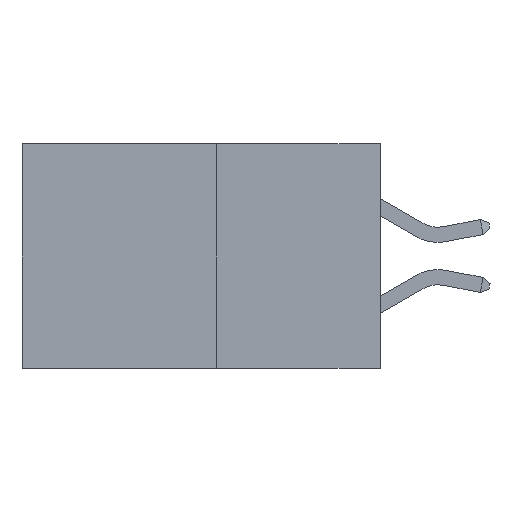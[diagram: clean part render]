
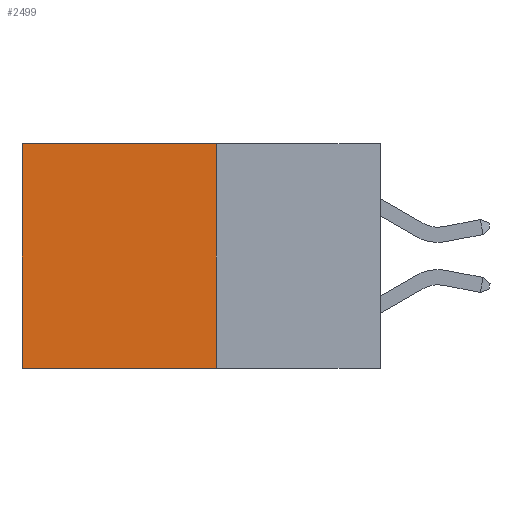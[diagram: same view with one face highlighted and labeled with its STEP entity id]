
A CAD part, left-side view. The second image highlights one B-rep face of the part: STEP entity #2499.
In plain terms, the highlighted planar face has unit normal (-1, 0, 0).
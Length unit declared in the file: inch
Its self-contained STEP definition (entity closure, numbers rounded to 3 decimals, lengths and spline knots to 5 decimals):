
#8 = LINE ( 'NONE', #19923, #23386 ) ;
#108 = CARTESIAN_POINT ( 'NONE',  ( 0.277, 0.59, 0. ) ) ;
#285 = VECTOR ( 'NONE', #12236, 39.37008 ) ;
#611 = ORIENTED_EDGE ( 'NONE', *, *, #14751, .T. ) ;
#1074 = CARTESIAN_POINT ( 'NONE',  ( 0.277, 0.59, -0.37 ) ) ;
#2183 = VERTEX_POINT ( 'NONE', #1074 ) ;
#2488 = ORIENTED_EDGE ( 'NONE', *, *, #27355, .T. ) ;
#2499 = ADVANCED_FACE ( 'NONE', ( #23911 ), #13537, .F. ) ;
#3717 = CARTESIAN_POINT ( 'NONE',  ( 0.277, 0.27, -0.37 ) ) ;
#5011 = DIRECTION ( 'NONE',  ( 0., 1., 0. ) ) ;
#6004 = EDGE_CURVE ( 'NONE', #26893, #2183, #6715, .T. ) ;
#6230 = CARTESIAN_POINT ( 'NONE',  ( 0.277, 0.27, -0.37 ) ) ;
#6715 = LINE ( 'NONE', #12341, #285 ) ;
#12236 = DIRECTION ( 'NONE',  ( 0., 1., 0. ) ) ;
#12341 = CARTESIAN_POINT ( 'NONE',  ( 0.277, 0.27, -0.37 ) ) ;
#13537 = PLANE ( 'NONE',  #23566 ) ;
#14751 = EDGE_CURVE ( 'NONE', #17969, #16574, #8, .T. ) ;
#16574 = VERTEX_POINT ( 'NONE', #108 ) ;
#16613 = ORIENTED_EDGE ( 'NONE', *, *, #6004, .F. ) ;
#17243 = LINE ( 'NONE', #24634, #17913 ) ;
#17913 = VECTOR ( 'NONE', #27132, 39.37008 ) ;
#17969 = VERTEX_POINT ( 'NONE', #21502 ) ;
#18850 = CARTESIAN_POINT ( 'NONE',  ( 0.277, 0.27, -0.37 ) ) ;
#19675 = LINE ( 'NONE', #18850, #24667 ) ;
#19848 = EDGE_CURVE ( 'NONE', #17969, #26893, #19675, .T. ) ;
#19923 = CARTESIAN_POINT ( 'NONE',  ( 0.277, 0.27, 0. ) ) ;
#20799 = ORIENTED_EDGE ( 'NONE', *, *, #19848, .F. ) ;
#20919 = DIRECTION ( 'NONE',  ( 0., 0., -1. ) ) ;
#21502 = CARTESIAN_POINT ( 'NONE',  ( 0.277, 0.27, 0. ) ) ;
#22233 = DIRECTION ( 'NONE',  ( 0., 0., -1. ) ) ;
#23386 = VECTOR ( 'NONE', #5011, 39.37008 ) ;
#23566 = AXIS2_PLACEMENT_3D ( 'NONE', #3717, #27013, #22233 ) ;
#23911 = FACE_OUTER_BOUND ( 'NONE', #27299, .T. ) ;
#24634 = CARTESIAN_POINT ( 'NONE',  ( 0.277, 0.59, -0.37 ) ) ;
#24667 = VECTOR ( 'NONE', #20919, 39.37008 ) ;
#26893 = VERTEX_POINT ( 'NONE', #6230 ) ;
#27013 = DIRECTION ( 'NONE',  ( 1., 0., 0. ) ) ;
#27132 = DIRECTION ( 'NONE',  ( 0., 0., -1. ) ) ;
#27299 = EDGE_LOOP ( 'NONE', ( #2488, #16613, #20799, #611 ) ) ;
#27355 = EDGE_CURVE ( 'NONE', #16574, #2183, #17243, .T. ) ;
